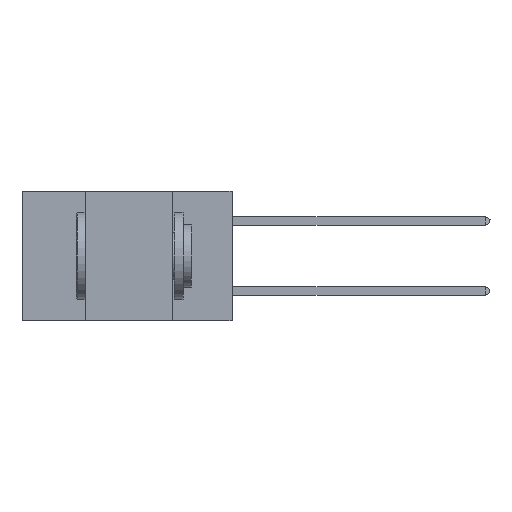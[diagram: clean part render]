
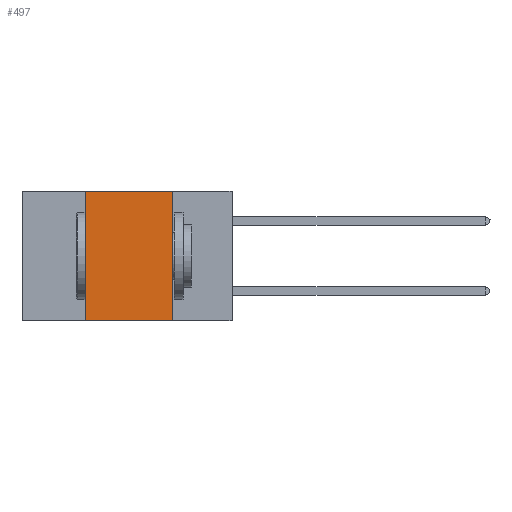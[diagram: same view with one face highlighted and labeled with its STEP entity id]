
A CAD part, left-side view. The second image highlights one B-rep face of the part: STEP entity #497.
In plain terms, the highlighted planar face has unit normal (-1, 0, 0).
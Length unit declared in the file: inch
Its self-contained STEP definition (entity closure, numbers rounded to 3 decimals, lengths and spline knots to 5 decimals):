
#497 = ADVANCED_FACE ( 'NONE', ( #17556 ), #19589, .F. ) ;
#608 = CARTESIAN_POINT ( 'NONE',  ( 0., 0.6, 0. ) ) ;
#1628 = CARTESIAN_POINT ( 'NONE',  ( 0., 0.6, 0. ) ) ;
#3485 = LINE ( 'NONE', #21981, #7560 ) ;
#4360 = VECTOR ( 'NONE', #19898, 39.37008 ) ;
#4638 = DIRECTION ( 'NONE',  ( 0., -1., 0. ) ) ;
#5754 = DIRECTION ( 'NONE',  ( 0., -1., 0. ) ) ;
#6782 = ORIENTED_EDGE ( 'NONE', *, *, #18966, .F. ) ;
#6818 = CARTESIAN_POINT ( 'NONE',  ( 0., 0.17, 0. ) ) ;
#7396 = ORIENTED_EDGE ( 'NONE', *, *, #15714, .T. ) ;
#7560 = VECTOR ( 'NONE', #5754, 39.37008 ) ;
#7652 = VERTEX_POINT ( 'NONE', #21389 ) ;
#8689 = CARTESIAN_POINT ( 'NONE',  ( 0., 0.42, 0. ) ) ;
#9853 = VECTOR ( 'NONE', #4638, 39.37008 ) ;
#9931 = ORIENTED_EDGE ( 'NONE', *, *, #16361, .F. ) ;
#10193 = ORIENTED_EDGE ( 'NONE', *, *, #15626, .F. ) ;
#11229 = CARTESIAN_POINT ( 'NONE',  ( 0., 0.17, 0. ) ) ;
#13548 = VERTEX_POINT ( 'NONE', #6818 ) ;
#15589 = DIRECTION ( 'NONE',  ( 0., 0., -1. ) ) ;
#15626 = EDGE_CURVE ( 'NONE', #13548, #25395, #21361, .T. ) ;
#15714 = EDGE_CURVE ( 'NONE', #19876, #25395, #3485, .T. ) ;
#15930 = CARTESIAN_POINT ( 'NONE',  ( 0., 0.42, -0.37 ) ) ;
#16361 = EDGE_CURVE ( 'NONE', #19876, #7652, #24817, .T. ) ;
#17556 = FACE_OUTER_BOUND ( 'NONE', #20369, .T. ) ;
#18477 = VECTOR ( 'NONE', #19314, 39.37008 ) ;
#18966 = EDGE_CURVE ( 'NONE', #7652, #13548, #21827, .T. ) ;
#19314 = DIRECTION ( 'NONE',  ( 0., 0., -1. ) ) ;
#19589 = PLANE ( 'NONE',  #20495 ) ;
#19717 = CARTESIAN_POINT ( 'NONE',  ( 0., 0.17, -0.37 ) ) ;
#19876 = VERTEX_POINT ( 'NONE', #15930 ) ;
#19898 = DIRECTION ( 'NONE',  ( 0., 0., 1. ) ) ;
#20369 = EDGE_LOOP ( 'NONE', ( #10193, #6782, #9931, #7396 ) ) ;
#20495 = AXIS2_PLACEMENT_3D ( 'NONE', #1628, #23931, #15589 ) ;
#21361 = LINE ( 'NONE', #11229, #18477 ) ;
#21389 = CARTESIAN_POINT ( 'NONE',  ( 0., 0.42, 0. ) ) ;
#21827 = LINE ( 'NONE', #608, #9853 ) ;
#21981 = CARTESIAN_POINT ( 'NONE',  ( 0., 0.6, -0.37 ) ) ;
#23931 = DIRECTION ( 'NONE',  ( 1., 0., 0. ) ) ;
#24817 = LINE ( 'NONE', #8689, #4360 ) ;
#25395 = VERTEX_POINT ( 'NONE', #19717 ) ;
